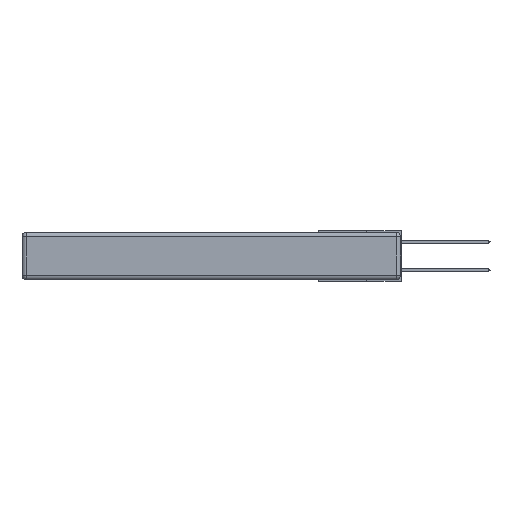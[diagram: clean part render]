
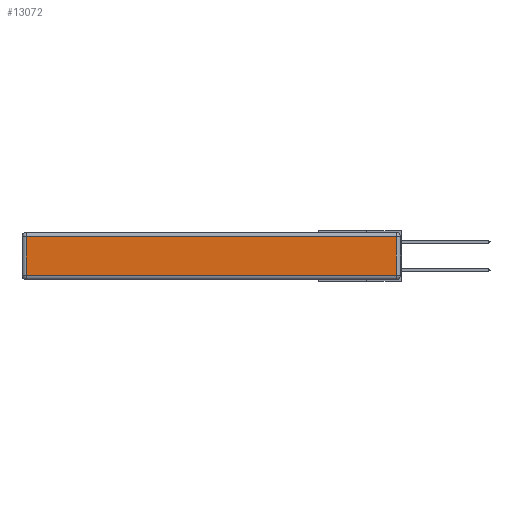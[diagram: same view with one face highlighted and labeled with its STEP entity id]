
A CAD part, left-side view. The second image highlights one B-rep face of the part: STEP entity #13072.
In plain terms, the highlighted planar face has unit normal (-1, 0, 0).
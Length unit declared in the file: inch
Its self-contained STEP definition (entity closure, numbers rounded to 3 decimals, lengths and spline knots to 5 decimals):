
#55 = EDGE_CURVE ( 'NONE', #4607, #17616, #13233, .T. ) ;
#1454 = CARTESIAN_POINT ( 'NONE',  ( 0., 2.75, -0.03 ) ) ;
#1788 = CARTESIAN_POINT ( 'NONE',  ( 0., 2.72, -0.343 ) ) ;
#2072 = CARTESIAN_POINT ( 'NONE',  ( 0., 0.03, -0.313 ) ) ;
#2523 = CARTESIAN_POINT ( 'NONE',  ( 0., 0., -0.313 ) ) ;
#3073 = VECTOR ( 'NONE', #5350, 39.37008 ) ;
#4607 = VERTEX_POINT ( 'NONE', #20170 ) ;
#5113 = LINE ( 'NONE', #2523, #13043 ) ;
#5183 = ORIENTED_EDGE ( 'NONE', *, *, #13025, .T. ) ;
#5283 = DIRECTION ( 'NONE',  ( -1., 0., 0. ) ) ;
#5350 = DIRECTION ( 'NONE',  ( 0., 0., 1. ) ) ;
#5596 = EDGE_LOOP ( 'NONE', ( #13365, #5183, #13590, #15044 ) ) ;
#5627 = FACE_OUTER_BOUND ( 'NONE', #5596, .T. ) ;
#6450 = VERTEX_POINT ( 'NONE', #2072 ) ;
#7084 = DIRECTION ( 'NONE',  ( 0., 0., 1. ) ) ;
#8423 = LINE ( 'NONE', #13352, #3073 ) ;
#8678 = EDGE_CURVE ( 'NONE', #15378, #6450, #5113, .T. ) ;
#9908 = EDGE_CURVE ( 'NONE', #17616, #15378, #19086, .T. ) ;
#10126 = CARTESIAN_POINT ( 'NONE',  ( 0., 0., -0.343 ) ) ;
#10495 = DIRECTION ( 'NONE',  ( 0., -1., 0. ) ) ;
#11919 = PLANE ( 'NONE',  #12373 ) ;
#12373 = AXIS2_PLACEMENT_3D ( 'NONE', #10126, #5283, #7084 ) ;
#12733 = VECTOR ( 'NONE', #16267, 39.37008 ) ;
#13025 = EDGE_CURVE ( 'NONE', #6450, #4607, #8423, .T. ) ;
#13043 = VECTOR ( 'NONE', #10495, 39.37008 ) ;
#13072 = ADVANCED_FACE ( 'NONE', ( #5627 ), #11919, .T. ) ;
#13233 = LINE ( 'NONE', #1454, #17301 ) ;
#13352 = CARTESIAN_POINT ( 'NONE',  ( 0., 0.03, -0.343 ) ) ;
#13365 = ORIENTED_EDGE ( 'NONE', *, *, #8678, .T. ) ;
#13590 = ORIENTED_EDGE ( 'NONE', *, *, #55, .T. ) ;
#14477 = CARTESIAN_POINT ( 'NONE',  ( 0., 2.72, -0.313 ) ) ;
#15044 = ORIENTED_EDGE ( 'NONE', *, *, #9908, .T. ) ;
#15378 = VERTEX_POINT ( 'NONE', #14477 ) ;
#16267 = DIRECTION ( 'NONE',  ( 0., 0., -1. ) ) ;
#17301 = VECTOR ( 'NONE', #17644, 39.37008 ) ;
#17616 = VERTEX_POINT ( 'NONE', #18966 ) ;
#17644 = DIRECTION ( 'NONE',  ( 0., 1., 0. ) ) ;
#18966 = CARTESIAN_POINT ( 'NONE',  ( 0., 2.72, -0.03 ) ) ;
#19086 = LINE ( 'NONE', #1788, #12733 ) ;
#20170 = CARTESIAN_POINT ( 'NONE',  ( 0., 0.03, -0.03 ) ) ;
